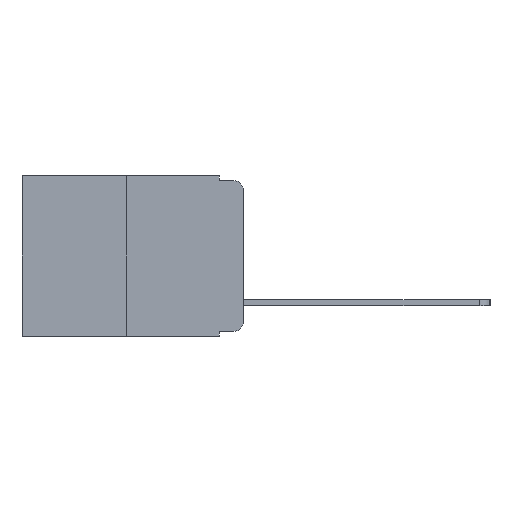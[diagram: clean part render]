
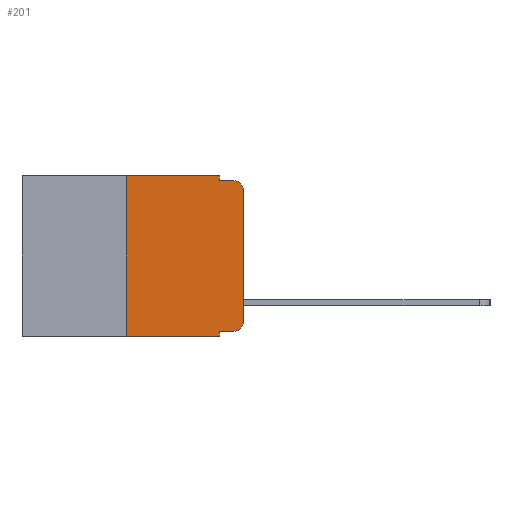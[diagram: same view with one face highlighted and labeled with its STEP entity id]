
A CAD part, left-side view. The second image highlights one B-rep face of the part: STEP entity #201.
In plain terms, the highlighted planar face has unit normal (-1, 0, 0).
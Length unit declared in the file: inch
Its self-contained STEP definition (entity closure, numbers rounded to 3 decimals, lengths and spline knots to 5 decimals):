
#79 = LINE ( 'NONE', #13630, #7319 ) ;
#178 = VERTEX_POINT ( 'NONE', #15144 ) ;
#201 = ADVANCED_FACE ( 'NONE', ( #12616 ), #16722, .F. ) ;
#236 = DIRECTION ( 'NONE',  ( 0., 0., 1. ) ) ;
#287 = VERTEX_POINT ( 'NONE', #8040 ) ;
#330 = LINE ( 'NONE', #16589, #5168 ) ;
#482 = CIRCLE ( 'NONE', #11363, 0.02 ) ;
#557 = CARTESIAN_POINT ( 'NONE',  ( 0., 0.051, 0. ) ) ;
#563 = EDGE_CURVE ( 'NONE', #3752, #287, #330, .T. ) ;
#688 = ORIENTED_EDGE ( 'NONE', *, *, #2563, .T. ) ;
#830 = DIRECTION ( 'NONE',  ( -1., 0., 0. ) ) ;
#898 = CARTESIAN_POINT ( 'NONE',  ( 0., 0.02, -0.03 ) ) ;
#1183 = CARTESIAN_POINT ( 'NONE',  ( 0., 0.25, 0. ) ) ;
#1184 = ORIENTED_EDGE ( 'NONE', *, *, #563, .F. ) ;
#1274 = VECTOR ( 'NONE', #7635, 39.37008 ) ;
#1854 = LINE ( 'NONE', #16792, #8914 ) ;
#2200 = VECTOR ( 'NONE', #13405, 39.37008 ) ;
#2563 = EDGE_CURVE ( 'NONE', #11805, #287, #482, .T. ) ;
#3021 = ORIENTED_EDGE ( 'NONE', *, *, #7684, .T. ) ;
#3356 = CARTESIAN_POINT ( 'NONE',  ( 0., 0.051, -0.333 ) ) ;
#3528 = EDGE_CURVE ( 'NONE', #10276, #11805, #4371, .T. ) ;
#3752 = VERTEX_POINT ( 'NONE', #17691 ) ;
#4168 = CARTESIAN_POINT ( 'NONE',  ( 0., 0.473, -0.343 ) ) ;
#4371 = LINE ( 'NONE', #9341, #8515 ) ;
#5168 = VECTOR ( 'NONE', #7740, 39.37008 ) ;
#5458 = VERTEX_POINT ( 'NONE', #7551 ) ;
#5597 = LINE ( 'NONE', #3356, #1274 ) ;
#6054 = CARTESIAN_POINT ( 'NONE',  ( 0., 0., -0.313 ) ) ;
#7018 = VERTEX_POINT ( 'NONE', #16183 ) ;
#7102 = CARTESIAN_POINT ( 'NONE',  ( 0., 0.02, -0.313 ) ) ;
#7209 = DIRECTION ( 'NONE',  ( 0., 0., -1. ) ) ;
#7319 = VECTOR ( 'NONE', #15002, 39.37008 ) ;
#7551 = CARTESIAN_POINT ( 'NONE',  ( 0., 0.051, -0.333 ) ) ;
#7628 = VERTEX_POINT ( 'NONE', #17414 ) ;
#7635 = DIRECTION ( 'NONE',  ( 0., -1., 0. ) ) ;
#7684 = EDGE_CURVE ( 'NONE', #7018, #10276, #17203, .T. ) ;
#7740 = DIRECTION ( 'NONE',  ( 0., -1., 0. ) ) ;
#8040 = CARTESIAN_POINT ( 'NONE',  ( 0., 0.02, -0.01 ) ) ;
#8337 = DIRECTION ( 'NONE',  ( 0., -1., 0. ) ) ;
#8484 = DIRECTION ( 'NONE',  ( 0., 0., -1. ) ) ;
#8515 = VECTOR ( 'NONE', #236, 39.37008 ) ;
#8584 = EDGE_CURVE ( 'NONE', #5458, #7018, #5597, .T. ) ;
#8774 = DIRECTION ( 'NONE',  ( 0., 0., -1. ) ) ;
#8914 = VECTOR ( 'NONE', #8774, 39.37008 ) ;
#9091 = LINE ( 'NONE', #1183, #12276 ) ;
#9132 = ORIENTED_EDGE ( 'NONE', *, *, #17534, .F. ) ;
#9179 = AXIS2_PLACEMENT_3D ( 'NONE', #15931, #16793, #16669 ) ;
#9238 = EDGE_LOOP ( 'NONE', ( #11464, #688, #1184, #9132, #12707, #13131, #16689, #13561, #17096, #3021 ) ) ;
#9341 = CARTESIAN_POINT ( 'NONE',  ( 0., 0., 0. ) ) ;
#9630 = DIRECTION ( 'NONE',  ( 0., 0., 1. ) ) ;
#10037 = CARTESIAN_POINT ( 'NONE',  ( 0., 0.25, 0. ) ) ;
#10276 = VERTEX_POINT ( 'NONE', #6054 ) ;
#10438 = CARTESIAN_POINT ( 'NONE',  ( 0., 0., -0.03 ) ) ;
#10736 = CARTESIAN_POINT ( 'NONE',  ( 0., 0.473, 0. ) ) ;
#11363 = AXIS2_PLACEMENT_3D ( 'NONE', #898, #830, #7209 ) ;
#11464 = ORIENTED_EDGE ( 'NONE', *, *, #3528, .T. ) ;
#11805 = VERTEX_POINT ( 'NONE', #10438 ) ;
#12218 = EDGE_CURVE ( 'NONE', #5458, #7628, #1854, .T. ) ;
#12276 = VECTOR ( 'NONE', #9630, 39.37008 ) ;
#12616 = FACE_OUTER_BOUND ( 'NONE', #9238, .T. ) ;
#12707 = ORIENTED_EDGE ( 'NONE', *, *, #15037, .F. ) ;
#13131 = ORIENTED_EDGE ( 'NONE', *, *, #15794, .F. ) ;
#13314 = EDGE_CURVE ( 'NONE', #178, #7628, #17250, .T. ) ;
#13405 = DIRECTION ( 'NONE',  ( 0., -1., 0. ) ) ;
#13561 = ORIENTED_EDGE ( 'NONE', *, *, #12218, .F. ) ;
#13630 = CARTESIAN_POINT ( 'NONE',  ( 0., 0.051, 0. ) ) ;
#13664 = LINE ( 'NONE', #10736, #2200 ) ;
#13698 = VERTEX_POINT ( 'NONE', #557 ) ;
#14160 = VECTOR ( 'NONE', #8337, 39.37008 ) ;
#15002 = DIRECTION ( 'NONE',  ( 0., 0., -1. ) ) ;
#15037 = EDGE_CURVE ( 'NONE', #15942, #13698, #13664, .T. ) ;
#15144 = CARTESIAN_POINT ( 'NONE',  ( 0., 0.25, -0.343 ) ) ;
#15794 = EDGE_CURVE ( 'NONE', #178, #15942, #9091, .T. ) ;
#15931 = CARTESIAN_POINT ( 'NONE',  ( 0., 0.473, 0. ) ) ;
#15942 = VERTEX_POINT ( 'NONE', #10037 ) ;
#16183 = CARTESIAN_POINT ( 'NONE',  ( 0., 0.02, -0.333 ) ) ;
#16502 = DIRECTION ( 'NONE',  ( -1., 0., 0. ) ) ;
#16589 = CARTESIAN_POINT ( 'NONE',  ( 0., 0.051, -0.01 ) ) ;
#16669 = DIRECTION ( 'NONE',  ( 0., 0., -1. ) ) ;
#16689 = ORIENTED_EDGE ( 'NONE', *, *, #13314, .T. ) ;
#16722 = PLANE ( 'NONE',  #9179 ) ;
#16792 = CARTESIAN_POINT ( 'NONE',  ( 0., 0.051, 0. ) ) ;
#16793 = DIRECTION ( 'NONE',  ( 1., 0., 0. ) ) ;
#17096 = ORIENTED_EDGE ( 'NONE', *, *, #8584, .T. ) ;
#17203 = CIRCLE ( 'NONE', #17635, 0.02 ) ;
#17250 = LINE ( 'NONE', #4168, #14160 ) ;
#17414 = CARTESIAN_POINT ( 'NONE',  ( 0., 0.051, -0.343 ) ) ;
#17534 = EDGE_CURVE ( 'NONE', #13698, #3752, #79, .T. ) ;
#17635 = AXIS2_PLACEMENT_3D ( 'NONE', #7102, #16502, #8484 ) ;
#17691 = CARTESIAN_POINT ( 'NONE',  ( 0., 0.051, -0.01 ) ) ;
